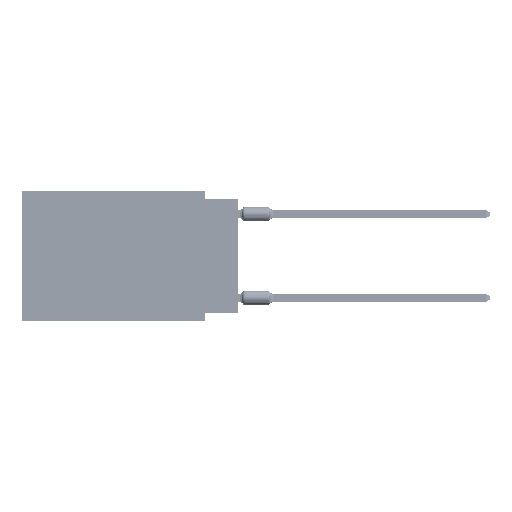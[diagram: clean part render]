
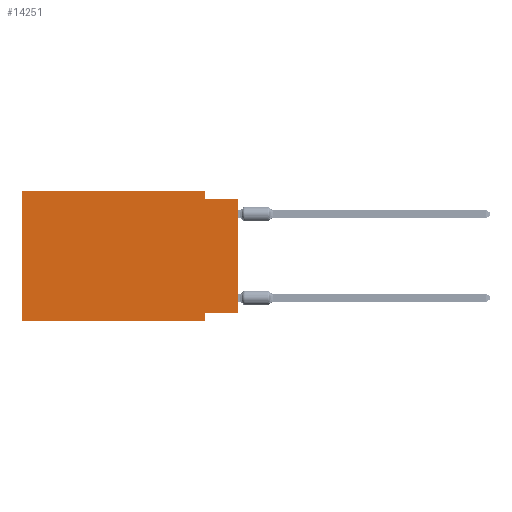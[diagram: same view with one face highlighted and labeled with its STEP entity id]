
A CAD part, left-side view. The second image highlights one B-rep face of the part: STEP entity #14251.
In plain terms, the highlighted planar face has unit normal (-1, 0, 0).
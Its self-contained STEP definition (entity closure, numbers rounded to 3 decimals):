
#457 = CARTESIAN_POINT ( 'NONE',  ( 0., 0., -0.635 ) ) ;
#2434 = EDGE_CURVE ( 'NONE', #66333, #6296, #62780, .T. ) ;
#3308 = CARTESIAN_POINT ( 'NONE',  ( 0., 2.54, 0. ) ) ;
#4157 = LINE ( 'NONE', #33035, #62876 ) ;
#4932 = VECTOR ( 'NONE', #31584, 1000. ) ;
#6296 = VERTEX_POINT ( 'NONE', #457 ) ;
#7284 = ORIENTED_EDGE ( 'NONE', *, *, #66336, .T. ) ;
#7540 = VERTEX_POINT ( 'NONE', #3308 ) ;
#8988 = LINE ( 'NONE', #19395, #4932 ) ;
#9783 = EDGE_LOOP ( 'NONE', ( #41312, #40472, #52044, #62809, #40289, #7284, #27980, #62842 ) ) ;
#10315 = CARTESIAN_POINT ( 'NONE',  ( 0., 2.54, 0. ) ) ;
#11810 = CARTESIAN_POINT ( 'NONE',  ( 0., 2.54, -0.635 ) ) ;
#12120 = PLANE ( 'NONE',  #19449 ) ;
#14251 = ADVANCED_FACE ( 'NONE', ( #34717 ), #12120, .F. ) ;
#14588 = DIRECTION ( 'NONE',  ( 0., 1., 0. ) ) ;
#16569 = CARTESIAN_POINT ( 'NONE',  ( 0., 16.383, 0. ) ) ;
#16970 = DIRECTION ( 'NONE',  ( 0., 0., -1. ) ) ;
#19395 = CARTESIAN_POINT ( 'NONE',  ( 0., 0., 0. ) ) ;
#19449 = AXIS2_PLACEMENT_3D ( 'NONE', #16569, #68403, #67315 ) ;
#20692 = CARTESIAN_POINT ( 'NONE',  ( 0., 16.383, 0. ) ) ;
#22926 = LINE ( 'NONE', #72212, #64156 ) ;
#27980 = ORIENTED_EDGE ( 'NONE', *, *, #31654, .F. ) ;
#28199 = VERTEX_POINT ( 'NONE', #56255 ) ;
#29615 = CARTESIAN_POINT ( 'NONE',  ( 0., 2.54, -9.271 ) ) ;
#29872 = VERTEX_POINT ( 'NONE', #33960 ) ;
#31584 = DIRECTION ( 'NONE',  ( 0., 0., 1. ) ) ;
#31654 = EDGE_CURVE ( 'NONE', #62151, #28199, #33282, .T. ) ;
#32021 = VERTEX_POINT ( 'NONE', #43960 ) ;
#32537 = DIRECTION ( 'NONE',  ( 0., 0., 1. ) ) ;
#33035 = CARTESIAN_POINT ( 'NONE',  ( 0., 16.383, 0. ) ) ;
#33282 = LINE ( 'NONE', #39213, #48430 ) ;
#33960 = CARTESIAN_POINT ( 'NONE',  ( 0., 16.383, -9.906 ) ) ;
#34083 = EDGE_CURVE ( 'NONE', #62257, #7540, #4157, .T. ) ;
#34717 = FACE_OUTER_BOUND ( 'NONE', #9783, .T. ) ;
#37087 = EDGE_CURVE ( 'NONE', #7540, #66333, #60715, .T. ) ;
#37541 = CARTESIAN_POINT ( 'NONE',  ( 0., 0., -9.271 ) ) ;
#39213 = CARTESIAN_POINT ( 'NONE',  ( 0., 2.54, -9.906 ) ) ;
#40289 = ORIENTED_EDGE ( 'NONE', *, *, #69076, .F. ) ;
#40472 = ORIENTED_EDGE ( 'NONE', *, *, #2434, .F. ) ;
#41312 = ORIENTED_EDGE ( 'NONE', *, *, #47597, .T. ) ;
#42554 = CARTESIAN_POINT ( 'NONE',  ( 0., 16.383, 0. ) ) ;
#42734 = LINE ( 'NONE', #37541, #61425 ) ;
#43416 = DIRECTION ( 'NONE',  ( 0., -1., 0. ) ) ;
#43960 = CARTESIAN_POINT ( 'NONE',  ( 0., 0., -9.271 ) ) ;
#47597 = EDGE_CURVE ( 'NONE', #32021, #6296, #8988, .T. ) ;
#48430 = VECTOR ( 'NONE', #49968, 1000. ) ;
#49968 = DIRECTION ( 'NONE',  ( 0., 0., -1. ) ) ;
#51132 = VECTOR ( 'NONE', #16970, 1000. ) ;
#52044 = ORIENTED_EDGE ( 'NONE', *, *, #37087, .F. ) ;
#56255 = CARTESIAN_POINT ( 'NONE',  ( 0., 2.54, -9.906 ) ) ;
#57232 = CARTESIAN_POINT ( 'NONE',  ( 0., 0., -0.635 ) ) ;
#57589 = VECTOR ( 'NONE', #63510, 1000. ) ;
#59946 = LINE ( 'NONE', #20692, #65398 ) ;
#60715 = LINE ( 'NONE', #10315, #51132 ) ;
#61425 = VECTOR ( 'NONE', #14588, 1000. ) ;
#61822 = DIRECTION ( 'NONE',  ( 0., -1., 0. ) ) ;
#62151 = VERTEX_POINT ( 'NONE', #29615 ) ;
#62257 = VERTEX_POINT ( 'NONE', #42554 ) ;
#62780 = LINE ( 'NONE', #57232, #57589 ) ;
#62809 = ORIENTED_EDGE ( 'NONE', *, *, #34083, .F. ) ;
#62842 = ORIENTED_EDGE ( 'NONE', *, *, #63235, .F. ) ;
#62876 = VECTOR ( 'NONE', #43416, 1000. ) ;
#63235 = EDGE_CURVE ( 'NONE', #32021, #62151, #42734, .T. ) ;
#63510 = DIRECTION ( 'NONE',  ( 0., -1., 0. ) ) ;
#64156 = VECTOR ( 'NONE', #61822, 1000. ) ;
#65398 = VECTOR ( 'NONE', #32537, 1000. ) ;
#66333 = VERTEX_POINT ( 'NONE', #11810 ) ;
#66336 = EDGE_CURVE ( 'NONE', #29872, #28199, #22926, .T. ) ;
#67315 = DIRECTION ( 'NONE',  ( 0., 0., -1. ) ) ;
#68403 = DIRECTION ( 'NONE',  ( 1., 0., 0. ) ) ;
#69076 = EDGE_CURVE ( 'NONE', #29872, #62257, #59946, .T. ) ;
#72212 = CARTESIAN_POINT ( 'NONE',  ( 0., 16.383, -9.906 ) ) ;
